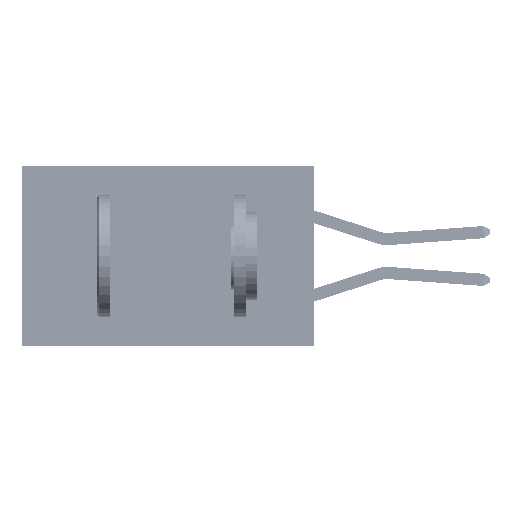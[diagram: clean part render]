
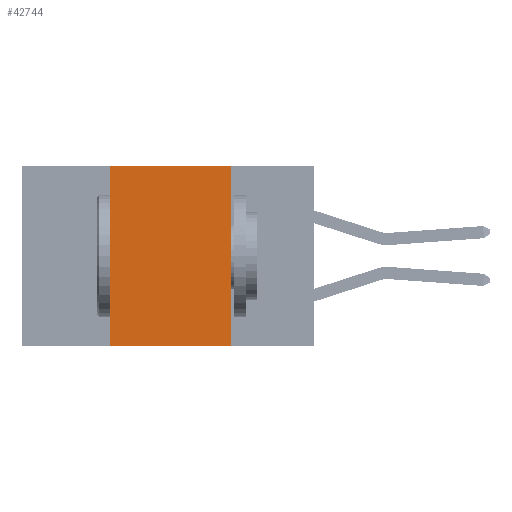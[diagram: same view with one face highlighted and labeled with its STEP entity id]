
A CAD part, left-side view. The second image highlights one B-rep face of the part: STEP entity #42744.
In plain terms, the highlighted planar face has unit normal (-1, 0, 0).
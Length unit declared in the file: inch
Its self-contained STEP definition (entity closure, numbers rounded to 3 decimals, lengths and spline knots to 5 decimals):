
#779 = CARTESIAN_POINT ( 'NONE',  ( 0., 0.6, 0. ) ) ;
#803 = ORIENTED_EDGE ( 'NONE', *, *, #25455, .F. ) ;
#1254 = LINE ( 'NONE', #41252, #39760 ) ;
#1975 = CARTESIAN_POINT ( 'NONE',  ( 0., 0.42, 0. ) ) ;
#4313 = DIRECTION ( 'NONE',  ( 1., 0., 0. ) ) ;
#4533 = EDGE_CURVE ( 'NONE', #35278, #41332, #6333, .T. ) ;
#4931 = PLANE ( 'NONE',  #22406 ) ;
#5790 = ORIENTED_EDGE ( 'NONE', *, *, #29676, .F. ) ;
#6333 = LINE ( 'NONE', #39589, #26118 ) ;
#7574 = FACE_OUTER_BOUND ( 'NONE', #24301, .T. ) ;
#9761 = VECTOR ( 'NONE', #13344, 39.37008 ) ;
#10241 = CARTESIAN_POINT ( 'NONE',  ( 0., 0.42, -0.37 ) ) ;
#12705 = ORIENTED_EDGE ( 'NONE', *, *, #4533, .T. ) ;
#13344 = DIRECTION ( 'NONE',  ( 0., 0., 1. ) ) ;
#13874 = CARTESIAN_POINT ( 'NONE',  ( 0., 0.17, 0. ) ) ;
#14302 = EDGE_CURVE ( 'NONE', #35278, #34652, #30133, .T. ) ;
#18036 = LINE ( 'NONE', #40056, #29036 ) ;
#18823 = DIRECTION ( 'NONE',  ( 0., -1., 0. ) ) ;
#22406 = AXIS2_PLACEMENT_3D ( 'NONE', #779, #4313, #29536 ) ;
#24301 = EDGE_LOOP ( 'NONE', ( #803, #5790, #24911, #12705 ) ) ;
#24911 = ORIENTED_EDGE ( 'NONE', *, *, #14302, .F. ) ;
#25455 = EDGE_CURVE ( 'NONE', #25551, #41332, #1254, .T. ) ;
#25551 = VERTEX_POINT ( 'NONE', #13874 ) ;
#26118 = VECTOR ( 'NONE', #18823, 39.37008 ) ;
#27256 = DIRECTION ( 'NONE',  ( 0., 0., -1. ) ) ;
#28100 = CARTESIAN_POINT ( 'NONE',  ( 0., 0.17, -0.37 ) ) ;
#29036 = VECTOR ( 'NONE', #36512, 39.37008 ) ;
#29536 = DIRECTION ( 'NONE',  ( 0., 0., -1. ) ) ;
#29676 = EDGE_CURVE ( 'NONE', #34652, #25551, #18036, .T. ) ;
#30133 = LINE ( 'NONE', #31034, #9761 ) ;
#31034 = CARTESIAN_POINT ( 'NONE',  ( 0., 0.42, 0. ) ) ;
#34652 = VERTEX_POINT ( 'NONE', #1975 ) ;
#35278 = VERTEX_POINT ( 'NONE', #10241 ) ;
#36512 = DIRECTION ( 'NONE',  ( 0., -1., 0. ) ) ;
#39589 = CARTESIAN_POINT ( 'NONE',  ( 0., 0.6, -0.37 ) ) ;
#39760 = VECTOR ( 'NONE', #27256, 39.37008 ) ;
#40056 = CARTESIAN_POINT ( 'NONE',  ( 0., 0.6, 0. ) ) ;
#41252 = CARTESIAN_POINT ( 'NONE',  ( 0., 0.17, 0. ) ) ;
#41332 = VERTEX_POINT ( 'NONE', #28100 ) ;
#42744 = ADVANCED_FACE ( 'NONE', ( #7574 ), #4931, .F. ) ;
